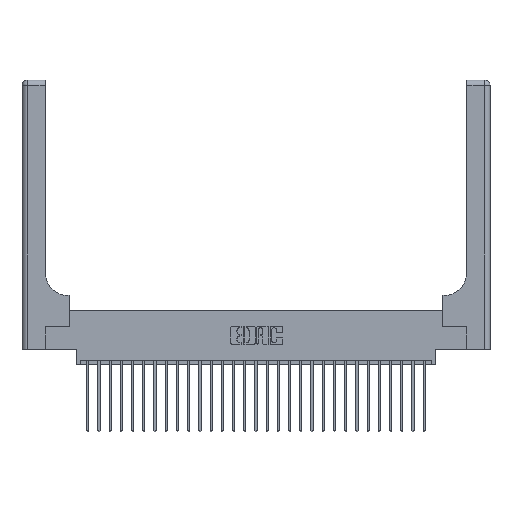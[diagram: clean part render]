
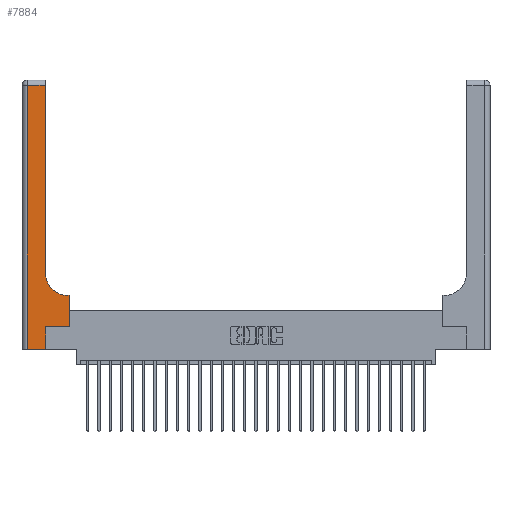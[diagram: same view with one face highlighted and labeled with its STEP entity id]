
A CAD part, top view. The second image highlights one B-rep face of the part: STEP entity #7884.
In plain terms, the highlighted planar face has unit normal (0, 0, 1).
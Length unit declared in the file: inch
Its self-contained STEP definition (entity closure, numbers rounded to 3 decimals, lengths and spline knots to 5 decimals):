
#104 = EDGE_CURVE ( 'NONE', #9318, #12331, #18252, .T. ) ;
#220 = CARTESIAN_POINT ( 'NONE',  ( 0.51, 0.85, 0.37 ) ) ;
#504 = VERTEX_POINT ( 'NONE', #19550 ) ;
#1214 = CARTESIAN_POINT ( 'NONE',  ( 0.528, 0.6, 0.37 ) ) ;
#1255 = VERTEX_POINT ( 'NONE', #1409 ) ;
#1409 = CARTESIAN_POINT ( 'NONE',  ( 0.51, 0.6, 0.37 ) ) ;
#1413 = DIRECTION ( 'NONE',  ( -1., 0., 0. ) ) ;
#2507 = CARTESIAN_POINT ( 'NONE',  ( 0.265, 0.25, 0.37 ) ) ;
#3935 = AXIS2_PLACEMENT_3D ( 'NONE', #220, #21110, #25555 ) ;
#4478 = ORIENTED_EDGE ( 'NONE', *, *, #14141, .T. ) ;
#4528 = EDGE_CURVE ( 'NONE', #1255, #9318, #15941, .T. ) ;
#4749 = ORIENTED_EDGE ( 'NONE', *, *, #21509, .T. ) ;
#4780 = EDGE_LOOP ( 'NONE', ( #24450, #5422, #4749, #26866, #25912, #16932, #16255, #4478, #5378 ) ) ;
#5378 = ORIENTED_EDGE ( 'NONE', *, *, #4528, .T. ) ;
#5422 = ORIENTED_EDGE ( 'NONE', *, *, #21931, .T. ) ;
#5729 = DIRECTION ( 'NONE',  ( 0., 1., 0. ) ) ;
#7220 = EDGE_CURVE ( 'NONE', #8331, #25059, #13489, .T. ) ;
#7348 = EDGE_CURVE ( 'NONE', #16751, #504, #17812, .T. ) ;
#7872 = FACE_OUTER_BOUND ( 'NONE', #4780, .T. ) ;
#7884 = ADVANCED_FACE ( 'NONE', ( #7872 ), #25271, .F. ) ;
#7946 = LINE ( 'NONE', #16310, #21601 ) ;
#8331 = VERTEX_POINT ( 'NONE', #20798 ) ;
#8966 = LINE ( 'NONE', #14960, #19883 ) ;
#9318 = VERTEX_POINT ( 'NONE', #26723 ) ;
#9436 = DIRECTION ( 'NONE',  ( -1., 0., 0. ) ) ;
#9882 = DIRECTION ( 'NONE',  ( 0., 1., 0. ) ) ;
#10335 = DIRECTION ( 'NONE',  ( 0., 1., 0. ) ) ;
#10359 = VECTOR ( 'NONE', #10335, 39.37008 ) ;
#10468 = LINE ( 'NONE', #27195, #10359 ) ;
#10500 = DIRECTION ( 'NONE',  ( 0., 0., -1. ) ) ;
#11967 = LINE ( 'NONE', #20487, #19672 ) ;
#12331 = VERTEX_POINT ( 'NONE', #24100 ) ;
#13489 = LINE ( 'NONE', #2507, #21773 ) ;
#14044 = CARTESIAN_POINT ( 'NONE',  ( 0., 0., 0.37 ) ) ;
#14049 = VECTOR ( 'NONE', #9882, 39.37008 ) ;
#14141 = EDGE_CURVE ( 'NONE', #20400, #1255, #11967, .T. ) ;
#14553 = CARTESIAN_POINT ( 'NONE',  ( 0.528, 0.25, 0.37 ) ) ;
#14779 = EDGE_CURVE ( 'NONE', #504, #8331, #10468, .T. ) ;
#14960 = CARTESIAN_POINT ( 'NONE',  ( 0.06, 3., 0.37 ) ) ;
#15432 = VECTOR ( 'NONE', #9436, 39.37008 ) ;
#15941 = CIRCLE ( 'NONE', #3935, 0.25 ) ;
#15982 = CARTESIAN_POINT ( 'NONE',  ( 0., 2.94, 0.37 ) ) ;
#16255 = ORIENTED_EDGE ( 'NONE', *, *, #19652, .T. ) ;
#16310 = CARTESIAN_POINT ( 'NONE',  ( 0.528, 0.25, 0.37 ) ) ;
#16751 = VERTEX_POINT ( 'NONE', #21722 ) ;
#16932 = ORIENTED_EDGE ( 'NONE', *, *, #7220, .T. ) ;
#16950 = CARTESIAN_POINT ( 'NONE',  ( 0.06, 2.94, 0.37 ) ) ;
#17767 = AXIS2_PLACEMENT_3D ( 'NONE', #20822, #10500, #18876 ) ;
#17812 = LINE ( 'NONE', #14044, #23996 ) ;
#18252 = LINE ( 'NONE', #22851, #14049 ) ;
#18870 = VERTEX_POINT ( 'NONE', #16950 ) ;
#18876 = DIRECTION ( 'NONE',  ( -1., 0., 0. ) ) ;
#19488 = DIRECTION ( 'NONE',  ( 1., 0., 0. ) ) ;
#19550 = CARTESIAN_POINT ( 'NONE',  ( 0.265, 0., 0.37 ) ) ;
#19652 = EDGE_CURVE ( 'NONE', #25059, #20400, #7946, .T. ) ;
#19672 = VECTOR ( 'NONE', #1413, 39.37008 ) ;
#19883 = VECTOR ( 'NONE', #23871, 39.37008 ) ;
#20400 = VERTEX_POINT ( 'NONE', #1214 ) ;
#20487 = CARTESIAN_POINT ( 'NONE',  ( 0.26, 0.6, 0.37 ) ) ;
#20798 = CARTESIAN_POINT ( 'NONE',  ( 0.265, 0.25, 0.37 ) ) ;
#20822 = CARTESIAN_POINT ( 'NONE',  ( 0., 3., 0.37 ) ) ;
#21110 = DIRECTION ( 'NONE',  ( 0., 0., -1. ) ) ;
#21509 = EDGE_CURVE ( 'NONE', #18870, #16751, #8966, .T. ) ;
#21601 = VECTOR ( 'NONE', #5729, 39.37008 ) ;
#21722 = CARTESIAN_POINT ( 'NONE',  ( 0.06, 0., 0.37 ) ) ;
#21773 = VECTOR ( 'NONE', #19488, 39.37008 ) ;
#21931 = EDGE_CURVE ( 'NONE', #12331, #18870, #26707, .T. ) ;
#22409 = DIRECTION ( 'NONE',  ( 1., 0., 0. ) ) ;
#22851 = CARTESIAN_POINT ( 'NONE',  ( 0.26, 3., 0.37 ) ) ;
#23871 = DIRECTION ( 'NONE',  ( 0., -1., 0. ) ) ;
#23996 = VECTOR ( 'NONE', #22409, 39.37008 ) ;
#24100 = CARTESIAN_POINT ( 'NONE',  ( 0.26, 2.94, 0.37 ) ) ;
#24450 = ORIENTED_EDGE ( 'NONE', *, *, #104, .T. ) ;
#25059 = VERTEX_POINT ( 'NONE', #14553 ) ;
#25271 = PLANE ( 'NONE',  #17767 ) ;
#25555 = DIRECTION ( 'NONE',  ( 1., 0., 0. ) ) ;
#25912 = ORIENTED_EDGE ( 'NONE', *, *, #14779, .T. ) ;
#26707 = LINE ( 'NONE', #15982, #15432 ) ;
#26723 = CARTESIAN_POINT ( 'NONE',  ( 0.26, 0.85, 0.37 ) ) ;
#26866 = ORIENTED_EDGE ( 'NONE', *, *, #7348, .T. ) ;
#27195 = CARTESIAN_POINT ( 'NONE',  ( 0.265, 0., 0.37 ) ) ;
